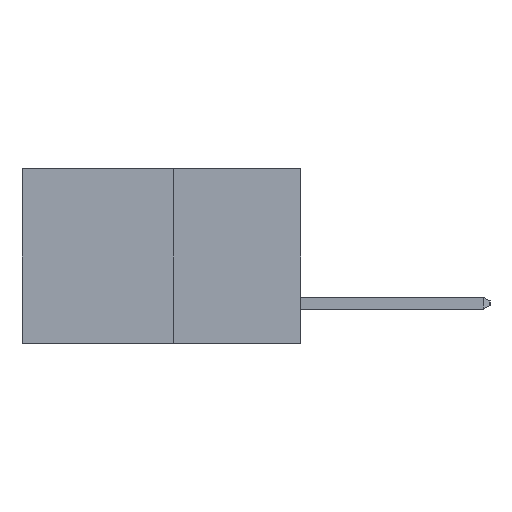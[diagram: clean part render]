
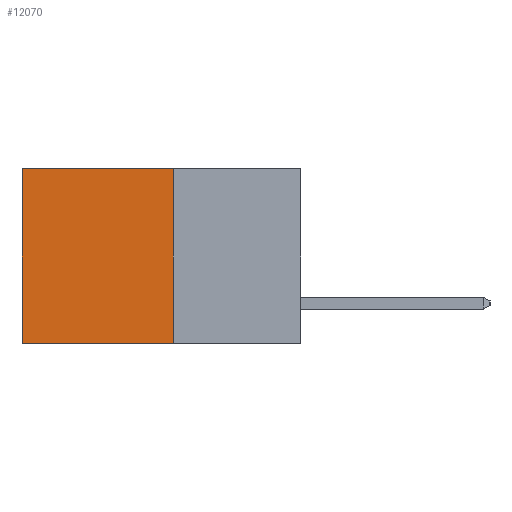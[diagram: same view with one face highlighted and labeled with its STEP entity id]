
A CAD part, left-side view. The second image highlights one B-rep face of the part: STEP entity #12070.
In plain terms, the highlighted planar face has unit normal (-1, 0, 0).
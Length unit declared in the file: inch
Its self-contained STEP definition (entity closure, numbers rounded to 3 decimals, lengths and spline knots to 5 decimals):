
#380 = DIRECTION ( 'NONE',  ( 1., 0., 0. ) ) ;
#566 = EDGE_CURVE ( 'NONE', #4126, #12464, #1713, .T. ) ;
#716 = AXIS2_PLACEMENT_3D ( 'NONE', #6397, #380, #8672 ) ;
#1069 = VECTOR ( 'NONE', #8057, 39.37008 ) ;
#1375 = ORIENTED_EDGE ( 'NONE', *, *, #14716, .T. ) ;
#1713 = LINE ( 'NONE', #3460, #4515 ) ;
#2947 = DIRECTION ( 'NONE',  ( 0., 0., -1. ) ) ;
#2959 = VECTOR ( 'NONE', #2947, 39.37008 ) ;
#3445 = EDGE_LOOP ( 'NONE', ( #1375, #4934, #8065, #8761 ) ) ;
#3460 = CARTESIAN_POINT ( 'NONE',  ( 0.277, 0.27, -0.37 ) ) ;
#3880 = DIRECTION ( 'NONE',  ( 0., 1., 0. ) ) ;
#4126 = VERTEX_POINT ( 'NONE', #13680 ) ;
#4515 = VECTOR ( 'NONE', #7876, 39.37008 ) ;
#4934 = ORIENTED_EDGE ( 'NONE', *, *, #10679, .F. ) ;
#5692 = FACE_OUTER_BOUND ( 'NONE', #3445, .T. ) ;
#6134 = CARTESIAN_POINT ( 'NONE',  ( 0.277, 0.59, 0. ) ) ;
#6171 = VERTEX_POINT ( 'NONE', #6134 ) ;
#6397 = CARTESIAN_POINT ( 'NONE',  ( 0.277, 0.27, -0.37 ) ) ;
#6913 = CARTESIAN_POINT ( 'NONE',  ( 0.277, 0.27, -0.37 ) ) ;
#7556 = PLANE ( 'NONE',  #716 ) ;
#7876 = DIRECTION ( 'NONE',  ( 0., 0., -1. ) ) ;
#8057 = DIRECTION ( 'NONE',  ( 0., 1., 0. ) ) ;
#8065 = ORIENTED_EDGE ( 'NONE', *, *, #566, .F. ) ;
#8074 = CARTESIAN_POINT ( 'NONE',  ( 0.277, 0.59, -0.37 ) ) ;
#8135 = EDGE_CURVE ( 'NONE', #4126, #6171, #10413, .T. ) ;
#8167 = VERTEX_POINT ( 'NONE', #9738 ) ;
#8276 = CARTESIAN_POINT ( 'NONE',  ( 0.277, 0.27, -0.37 ) ) ;
#8672 = DIRECTION ( 'NONE',  ( 0., 0., -1. ) ) ;
#8761 = ORIENTED_EDGE ( 'NONE', *, *, #8135, .T. ) ;
#9733 = VECTOR ( 'NONE', #3880, 39.37008 ) ;
#9738 = CARTESIAN_POINT ( 'NONE',  ( 0.277, 0.59, -0.37 ) ) ;
#10353 = LINE ( 'NONE', #6913, #1069 ) ;
#10413 = LINE ( 'NONE', #11804, #9733 ) ;
#10679 = EDGE_CURVE ( 'NONE', #12464, #8167, #10353, .T. ) ;
#11804 = CARTESIAN_POINT ( 'NONE',  ( 0.277, 0.27, 0. ) ) ;
#12070 = ADVANCED_FACE ( 'NONE', ( #5692 ), #7556, .F. ) ;
#12464 = VERTEX_POINT ( 'NONE', #8276 ) ;
#12712 = LINE ( 'NONE', #8074, #2959 ) ;
#13680 = CARTESIAN_POINT ( 'NONE',  ( 0.277, 0.27, 0. ) ) ;
#14716 = EDGE_CURVE ( 'NONE', #6171, #8167, #12712, .T. ) ;
